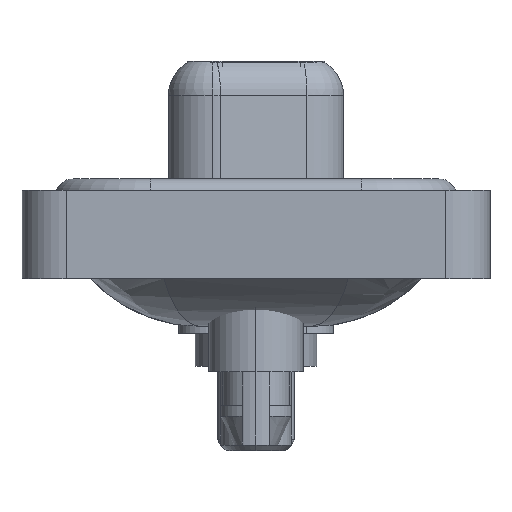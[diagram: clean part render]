
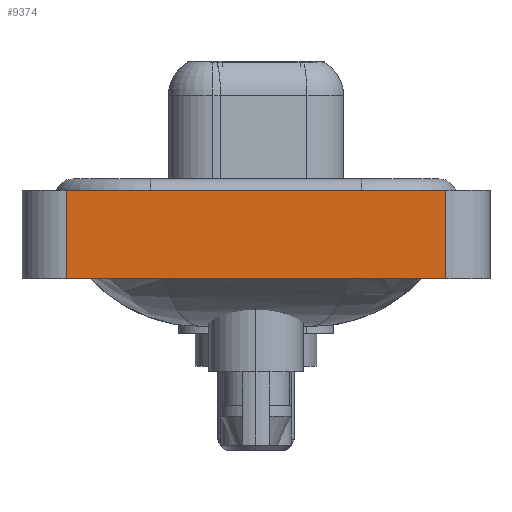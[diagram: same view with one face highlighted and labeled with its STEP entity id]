
A CAD part, left-side view. The second image highlights one B-rep face of the part: STEP entity #9374.
In plain terms, the highlighted planar face has unit normal (-1, 0, 0).
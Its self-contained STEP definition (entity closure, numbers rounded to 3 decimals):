
#331 = ORIENTED_EDGE ( 'NONE', *, *, #20559, .T. ) ;
#777 = VERTEX_POINT ( 'NONE', #11896 ) ;
#1405 = DIRECTION ( 'NONE',  ( 0., -1., 0. ) ) ;
#3540 = ORIENTED_EDGE ( 'NONE', *, *, #16491, .F. ) ;
#3686 = VERTEX_POINT ( 'NONE', #15842 ) ;
#4990 = CARTESIAN_POINT ( 'NONE',  ( -7.35, 8.55, -3.6 ) ) ;
#6151 = PLANE ( 'NONE',  #13788 ) ;
#6376 = DIRECTION ( 'NONE',  ( 0., 0., 1. ) ) ;
#6610 = CARTESIAN_POINT ( 'NONE',  ( -7.35, -8.55, 0.4 ) ) ;
#6713 = CARTESIAN_POINT ( 'NONE',  ( -7.35, -8.55, -3.6 ) ) ;
#6719 = CARTESIAN_POINT ( 'NONE',  ( -7.35, -8.55, 0.4 ) ) ;
#8451 = EDGE_LOOP ( 'NONE', ( #19176, #3540, #15836, #331 ) ) ;
#9138 = EDGE_CURVE ( 'NONE', #16382, #17925, #11224, .T. ) ;
#9308 = VECTOR ( 'NONE', #20947, 1000. ) ;
#9374 = ADVANCED_FACE ( 'NONE', ( #16677 ), #6151, .T. ) ;
#11136 = EDGE_CURVE ( 'NONE', #777, #3686, #20484, .T. ) ;
#11224 = LINE ( 'NONE', #21321, #20663 ) ;
#11463 = LINE ( 'NONE', #6610, #17184 ) ;
#11896 = CARTESIAN_POINT ( 'NONE',  ( -7.35, 8.55, -3.6 ) ) ;
#13033 = CARTESIAN_POINT ( 'NONE',  ( -7.35, -8.55, -3.6 ) ) ;
#13788 = AXIS2_PLACEMENT_3D ( 'NONE', #13033, #19946, #6376 ) ;
#14049 = CARTESIAN_POINT ( 'NONE',  ( -7.35, -8.55, -3.6 ) ) ;
#14191 = DIRECTION ( 'NONE',  ( 0., 0., 1. ) ) ;
#15678 = VECTOR ( 'NONE', #20594, 1000. ) ;
#15836 = ORIENTED_EDGE ( 'NONE', *, *, #11136, .F. ) ;
#15842 = CARTESIAN_POINT ( 'NONE',  ( -7.35, 8.55, 0.4 ) ) ;
#16382 = VERTEX_POINT ( 'NONE', #6713 ) ;
#16491 = EDGE_CURVE ( 'NONE', #3686, #17925, #11463, .T. ) ;
#16677 = FACE_OUTER_BOUND ( 'NONE', #8451, .T. ) ;
#17184 = VECTOR ( 'NONE', #1405, 1000. ) ;
#17444 = LINE ( 'NONE', #14049, #9308 ) ;
#17925 = VERTEX_POINT ( 'NONE', #6719 ) ;
#19176 = ORIENTED_EDGE ( 'NONE', *, *, #9138, .T. ) ;
#19946 = DIRECTION ( 'NONE',  ( -1., 0., 0. ) ) ;
#20484 = LINE ( 'NONE', #4990, #15678 ) ;
#20559 = EDGE_CURVE ( 'NONE', #777, #16382, #17444, .T. ) ;
#20594 = DIRECTION ( 'NONE',  ( 0., 0., 1. ) ) ;
#20663 = VECTOR ( 'NONE', #14191, 1000. ) ;
#20947 = DIRECTION ( 'NONE',  ( 0., -1., 0. ) ) ;
#21321 = CARTESIAN_POINT ( 'NONE',  ( -7.35, -8.55, -3.6 ) ) ;
